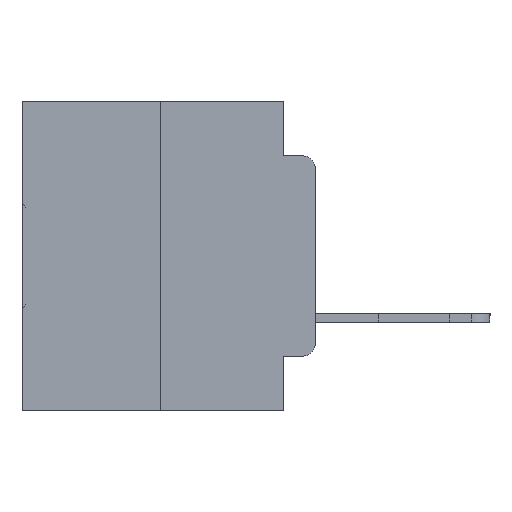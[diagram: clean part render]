
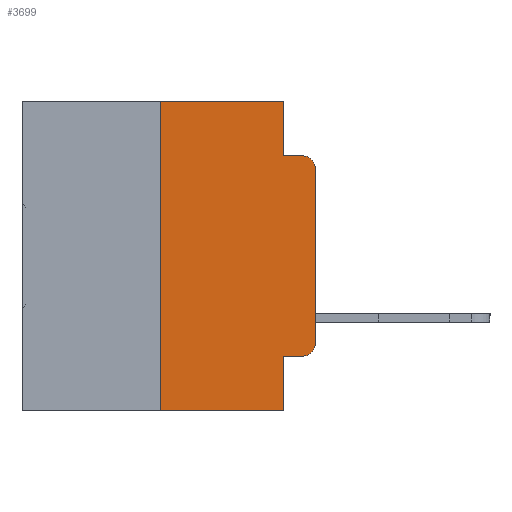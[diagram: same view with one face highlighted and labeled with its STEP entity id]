
A CAD part, left-side view. The second image highlights one B-rep face of the part: STEP entity #3699.
In plain terms, the highlighted planar face has unit normal (-1, 0, 0).
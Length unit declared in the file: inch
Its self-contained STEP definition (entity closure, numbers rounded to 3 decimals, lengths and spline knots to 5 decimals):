
#233 = ORIENTED_EDGE ( 'NONE', *, *, #15432, .F. ) ;
#394 = LINE ( 'NONE', #15305, #19592 ) ;
#679 = LINE ( 'NONE', #13027, #25491 ) ;
#780 = LINE ( 'NONE', #14504, #13515 ) ;
#1183 = LINE ( 'NONE', #17688, #26699 ) ;
#1353 = VECTOR ( 'NONE', #29972, 39.37008 ) ;
#2502 = CARTESIAN_POINT ( 'NONE',  ( 0., 0.25, -0.5 ) ) ;
#3678 = CARTESIAN_POINT ( 'NONE',  ( 0., 0.02, -0.1085 ) ) ;
#3699 = ADVANCED_FACE ( 'NONE', ( #27560 ), #30091, .F. ) ;
#4255 = ORIENTED_EDGE ( 'NONE', *, *, #21648, .T. ) ;
#4464 = CARTESIAN_POINT ( 'NONE',  ( 0., 0., -0.3915 ) ) ;
#4641 = VECTOR ( 'NONE', #26602, 39.37008 ) ;
#5095 = DIRECTION ( 'NONE',  ( 1., 0., 0. ) ) ;
#5399 = EDGE_CURVE ( 'NONE', #19726, #18641, #394, .T. ) ;
#5434 = LINE ( 'NONE', #12094, #4641 ) ;
#5500 = CARTESIAN_POINT ( 'NONE',  ( 0., 0.051, -0.4115 ) ) ;
#5984 = VERTEX_POINT ( 'NONE', #27430 ) ;
#6207 = DIRECTION ( 'NONE',  ( 0., 0., -1. ) ) ;
#6684 = CARTESIAN_POINT ( 'NONE',  ( 0., 0.473, -0.5 ) ) ;
#6700 = DIRECTION ( 'NONE',  ( -1., 0., 0. ) ) ;
#6848 = ORIENTED_EDGE ( 'NONE', *, *, #16395, .T. ) ;
#8341 = EDGE_CURVE ( 'NONE', #26053, #14491, #780, .T. ) ;
#10078 = ORIENTED_EDGE ( 'NONE', *, *, #25350, .T. ) ;
#10130 = ORIENTED_EDGE ( 'NONE', *, *, #5399, .T. ) ;
#12094 = CARTESIAN_POINT ( 'NONE',  ( 0., 0.051, -0.0885 ) ) ;
#12117 = ORIENTED_EDGE ( 'NONE', *, *, #16495, .F. ) ;
#12472 = VERTEX_POINT ( 'NONE', #19727 ) ;
#12801 = AXIS2_PLACEMENT_3D ( 'NONE', #3678, #20993, #6207 ) ;
#12806 = DIRECTION ( 'NONE',  ( 0., 0., 1. ) ) ;
#13027 = CARTESIAN_POINT ( 'NONE',  ( 0., 0.051, 0. ) ) ;
#13515 = VECTOR ( 'NONE', #19358, 39.37008 ) ;
#13658 = ORIENTED_EDGE ( 'NONE', *, *, #25986, .T. ) ;
#14300 = DIRECTION ( 'NONE',  ( 0., -1., 0. ) ) ;
#14491 = VERTEX_POINT ( 'NONE', #14897 ) ;
#14504 = CARTESIAN_POINT ( 'NONE',  ( 0., 0.473, 0. ) ) ;
#14530 = ORIENTED_EDGE ( 'NONE', *, *, #8341, .F. ) ;
#14897 = CARTESIAN_POINT ( 'NONE',  ( 0., 0.051, 0. ) ) ;
#15051 = CARTESIAN_POINT ( 'NONE',  ( 0., 0.051, -0.5 ) ) ;
#15305 = CARTESIAN_POINT ( 'NONE',  ( 0., 0., 0. ) ) ;
#15432 = EDGE_CURVE ( 'NONE', #28631, #26053, #30968, .T. ) ;
#15618 = CARTESIAN_POINT ( 'NONE',  ( 0., 0.051, -0.4115 ) ) ;
#15654 = ORIENTED_EDGE ( 'NONE', *, *, #27501, .F. ) ;
#15814 = VECTOR ( 'NONE', #14300, 39.37008 ) ;
#16378 = CARTESIAN_POINT ( 'NONE',  ( 0., 0.25, 0. ) ) ;
#16395 = EDGE_CURVE ( 'NONE', #20379, #19726, #27281, .T. ) ;
#16495 = EDGE_CURVE ( 'NONE', #12472, #5984, #5434, .T. ) ;
#17688 = CARTESIAN_POINT ( 'NONE',  ( 0., 0.051, 0. ) ) ;
#17973 = VERTEX_POINT ( 'NONE', #5500 ) ;
#18641 = VERTEX_POINT ( 'NONE', #21847 ) ;
#18840 = EDGE_CURVE ( 'NONE', #17973, #22107, #679, .T. ) ;
#19358 = DIRECTION ( 'NONE',  ( 0., -1., 0. ) ) ;
#19592 = VECTOR ( 'NONE', #12806, 39.37008 ) ;
#19726 = VERTEX_POINT ( 'NONE', #4464 ) ;
#19727 = CARTESIAN_POINT ( 'NONE',  ( 0., 0.051, -0.0885 ) ) ;
#20160 = DIRECTION ( 'NONE',  ( 0., 0., -1. ) ) ;
#20379 = VERTEX_POINT ( 'NONE', #26454 ) ;
#20993 = DIRECTION ( 'NONE',  ( -1., 0., 0. ) ) ;
#21246 = DIRECTION ( 'NONE',  ( 0., 0., 1. ) ) ;
#21481 = CARTESIAN_POINT ( 'NONE',  ( 0., 0.02, -0.3915 ) ) ;
#21648 = EDGE_CURVE ( 'NONE', #17973, #20379, #27568, .T. ) ;
#21847 = CARTESIAN_POINT ( 'NONE',  ( 0., 0., -0.1085 ) ) ;
#22107 = VERTEX_POINT ( 'NONE', #15051 ) ;
#22214 = LINE ( 'NONE', #6684, #15814 ) ;
#22260 = AXIS2_PLACEMENT_3D ( 'NONE', #22772, #5095, #20160 ) ;
#22772 = CARTESIAN_POINT ( 'NONE',  ( 0., 0.473, 0. ) ) ;
#23554 = CARTESIAN_POINT ( 'NONE',  ( 0., 0.25, 0. ) ) ;
#23876 = DIRECTION ( 'NONE',  ( 0., 0., -1. ) ) ;
#24752 = VECTOR ( 'NONE', #21246, 39.37008 ) ;
#25350 = EDGE_CURVE ( 'NONE', #28631, #22107, #22214, .T. ) ;
#25491 = VECTOR ( 'NONE', #29774, 39.37008 ) ;
#25986 = EDGE_CURVE ( 'NONE', #18641, #5984, #28857, .T. ) ;
#26053 = VERTEX_POINT ( 'NONE', #16378 ) ;
#26454 = CARTESIAN_POINT ( 'NONE',  ( 0., 0.02, -0.4115 ) ) ;
#26602 = DIRECTION ( 'NONE',  ( 0., -1., 0. ) ) ;
#26612 = EDGE_LOOP ( 'NONE', ( #10130, #13658, #12117, #15654, #14530, #233, #10078, #28858, #4255, #6848 ) ) ;
#26699 = VECTOR ( 'NONE', #27210, 39.37008 ) ;
#27174 = AXIS2_PLACEMENT_3D ( 'NONE', #21481, #6700, #23876 ) ;
#27210 = DIRECTION ( 'NONE',  ( 0., 0., -1. ) ) ;
#27281 = CIRCLE ( 'NONE', #27174, 0.02 ) ;
#27430 = CARTESIAN_POINT ( 'NONE',  ( 0., 0.02, -0.0885 ) ) ;
#27501 = EDGE_CURVE ( 'NONE', #14491, #12472, #1183, .T. ) ;
#27560 = FACE_OUTER_BOUND ( 'NONE', #26612, .T. ) ;
#27568 = LINE ( 'NONE', #15618, #1353 ) ;
#28631 = VERTEX_POINT ( 'NONE', #2502 ) ;
#28857 = CIRCLE ( 'NONE', #12801, 0.02 ) ;
#28858 = ORIENTED_EDGE ( 'NONE', *, *, #18840, .F. ) ;
#29774 = DIRECTION ( 'NONE',  ( 0., 0., -1. ) ) ;
#29972 = DIRECTION ( 'NONE',  ( 0., -1., 0. ) ) ;
#30091 = PLANE ( 'NONE',  #22260 ) ;
#30968 = LINE ( 'NONE', #23554, #24752 ) ;
